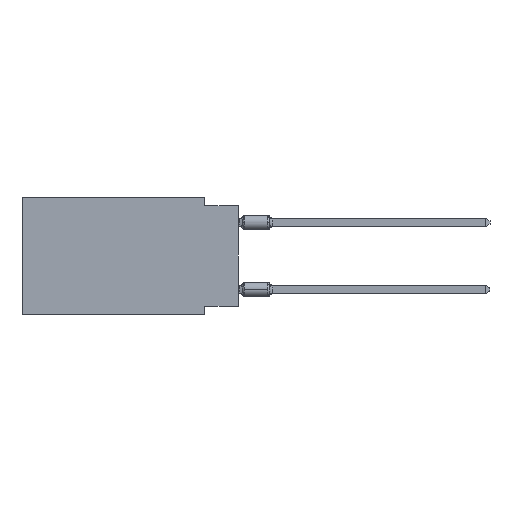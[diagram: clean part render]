
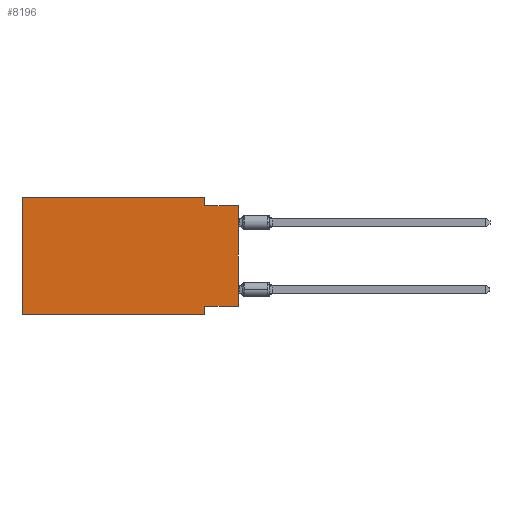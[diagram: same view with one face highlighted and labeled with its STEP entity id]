
A CAD part, left-side view. The second image highlights one B-rep face of the part: STEP entity #8196.
In plain terms, the highlighted planar face has unit normal (-1, 0, 0).
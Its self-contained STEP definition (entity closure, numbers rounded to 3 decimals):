
#128 = VECTOR ( 'NONE', #23519, 1000. ) ;
#239 = EDGE_CURVE ( 'NONE', #10833, #5757, #17624, .T. ) ;
#240 = EDGE_LOOP ( 'NONE', ( #4774, #21233, #8621, #17135, #16062, #23775, #12393, #20867 ) ) ;
#541 = LINE ( 'NONE', #12511, #3268 ) ;
#590 = EDGE_CURVE ( 'NONE', #22374, #4288, #6799, .T. ) ;
#746 = CARTESIAN_POINT ( 'NONE',  ( 0., 16.383, -8.89 ) ) ;
#871 = VECTOR ( 'NONE', #1895, 1000. ) ;
#1211 = CARTESIAN_POINT ( 'NONE',  ( 0., 2.54, 0. ) ) ;
#1895 = DIRECTION ( 'NONE',  ( 0., 0., -1. ) ) ;
#1913 = VERTEX_POINT ( 'NONE', #23687 ) ;
#3268 = VECTOR ( 'NONE', #16759, 1000. ) ;
#3677 = EDGE_CURVE ( 'NONE', #12716, #21977, #17557, .T. ) ;
#4007 = VECTOR ( 'NONE', #5197, 1000. ) ;
#4288 = VERTEX_POINT ( 'NONE', #5371 ) ;
#4395 = DIRECTION ( 'NONE',  ( 0., 0., -1. ) ) ;
#4774 = ORIENTED_EDGE ( 'NONE', *, *, #5066, .T. ) ;
#5066 = EDGE_CURVE ( 'NONE', #22374, #1913, #541, .T. ) ;
#5134 = DIRECTION ( 'NONE',  ( 0., 0., 1. ) ) ;
#5197 = DIRECTION ( 'NONE',  ( 0., 1., 0. ) ) ;
#5351 = AXIS2_PLACEMENT_3D ( 'NONE', #8897, #12377, #4395 ) ;
#5371 = CARTESIAN_POINT ( 'NONE',  ( 0., 2.54, -8.255 ) ) ;
#5757 = VERTEX_POINT ( 'NONE', #25594 ) ;
#6799 = LINE ( 'NONE', #23388, #4007 ) ;
#6850 = DIRECTION ( 'NONE',  ( 0., -1., 0. ) ) ;
#8196 = ADVANCED_FACE ( 'NONE', ( #18606 ), #22586, .F. ) ;
#8449 = VECTOR ( 'NONE', #23540, 1000. ) ;
#8621 = ORIENTED_EDGE ( 'NONE', *, *, #3677, .F. ) ;
#8683 = CARTESIAN_POINT ( 'NONE',  ( 0., 2.54, -0.635 ) ) ;
#8897 = CARTESIAN_POINT ( 'NONE',  ( 0., 16.383, 0. ) ) ;
#10429 = EDGE_CURVE ( 'NONE', #10833, #18518, #21451, .T. ) ;
#10833 = VERTEX_POINT ( 'NONE', #20901 ) ;
#11204 = LINE ( 'NONE', #17448, #8449 ) ;
#12377 = DIRECTION ( 'NONE',  ( 1., 0., 0. ) ) ;
#12393 = ORIENTED_EDGE ( 'NONE', *, *, #25088, .F. ) ;
#12511 = CARTESIAN_POINT ( 'NONE',  ( 0., 0., 0. ) ) ;
#12716 = VERTEX_POINT ( 'NONE', #1211 ) ;
#14439 = EDGE_CURVE ( 'NONE', #21977, #1913, #23623, .T. ) ;
#15109 = VECTOR ( 'NONE', #5134, 1000. ) ;
#15569 = CARTESIAN_POINT ( 'NONE',  ( 0., 2.54, -8.89 ) ) ;
#16062 = ORIENTED_EDGE ( 'NONE', *, *, #239, .F. ) ;
#16631 = CARTESIAN_POINT ( 'NONE',  ( 0., 0., -8.255 ) ) ;
#16759 = DIRECTION ( 'NONE',  ( 0., 0., 1. ) ) ;
#16953 = VECTOR ( 'NONE', #6850, 1000. ) ;
#17135 = ORIENTED_EDGE ( 'NONE', *, *, #19117, .F. ) ;
#17448 = CARTESIAN_POINT ( 'NONE',  ( 0., 2.54, -8.89 ) ) ;
#17557 = LINE ( 'NONE', #21940, #871 ) ;
#17624 = LINE ( 'NONE', #19353, #15109 ) ;
#18148 = VECTOR ( 'NONE', #25759, 1000. ) ;
#18518 = VERTEX_POINT ( 'NONE', #15569 ) ;
#18606 = FACE_OUTER_BOUND ( 'NONE', #240, .T. ) ;
#18927 = LINE ( 'NONE', #20911, #128 ) ;
#19117 = EDGE_CURVE ( 'NONE', #5757, #12716, #18927, .T. ) ;
#19353 = CARTESIAN_POINT ( 'NONE',  ( 0., 16.383, 0. ) ) ;
#20867 = ORIENTED_EDGE ( 'NONE', *, *, #590, .F. ) ;
#20901 = CARTESIAN_POINT ( 'NONE',  ( 0., 16.383, -8.89 ) ) ;
#20911 = CARTESIAN_POINT ( 'NONE',  ( 0., 16.383, 0. ) ) ;
#21233 = ORIENTED_EDGE ( 'NONE', *, *, #14439, .F. ) ;
#21451 = LINE ( 'NONE', #746, #16953 ) ;
#21639 = CARTESIAN_POINT ( 'NONE',  ( 0., 0., -0.635 ) ) ;
#21940 = CARTESIAN_POINT ( 'NONE',  ( 0., 2.54, 0. ) ) ;
#21977 = VERTEX_POINT ( 'NONE', #8683 ) ;
#22374 = VERTEX_POINT ( 'NONE', #16631 ) ;
#22586 = PLANE ( 'NONE',  #5351 ) ;
#23388 = CARTESIAN_POINT ( 'NONE',  ( 0., 0., -8.255 ) ) ;
#23519 = DIRECTION ( 'NONE',  ( 0., -1., 0. ) ) ;
#23540 = DIRECTION ( 'NONE',  ( 0., 0., -1. ) ) ;
#23623 = LINE ( 'NONE', #21639, #18148 ) ;
#23687 = CARTESIAN_POINT ( 'NONE',  ( 0., 0., -0.635 ) ) ;
#23775 = ORIENTED_EDGE ( 'NONE', *, *, #10429, .T. ) ;
#25088 = EDGE_CURVE ( 'NONE', #4288, #18518, #11204, .T. ) ;
#25594 = CARTESIAN_POINT ( 'NONE',  ( 0., 16.383, 0. ) ) ;
#25759 = DIRECTION ( 'NONE',  ( 0., -1., 0. ) ) ;
